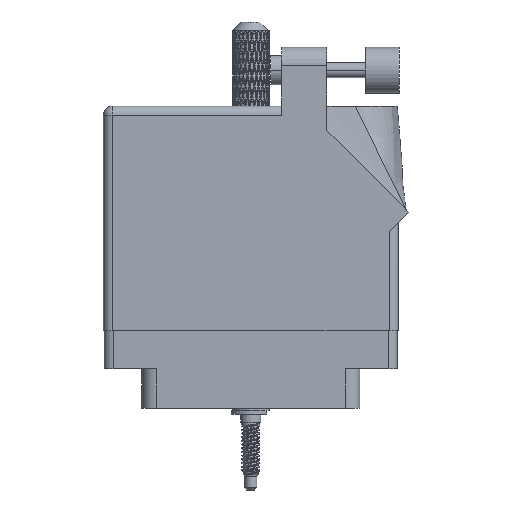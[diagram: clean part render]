
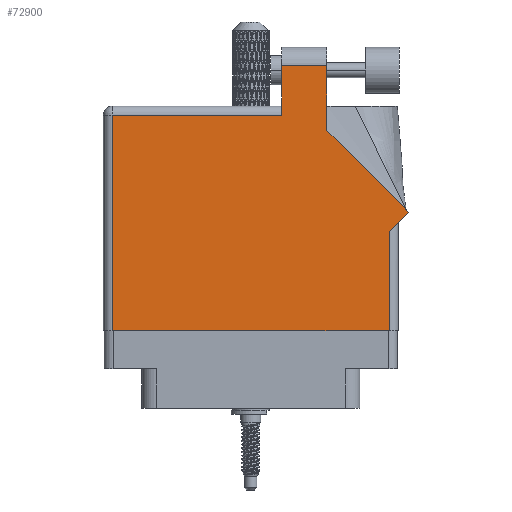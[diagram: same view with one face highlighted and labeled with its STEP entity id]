
A CAD part, front view. The second image highlights one B-rep face of the part: STEP entity #72900.
In plain terms, the highlighted face is planar.
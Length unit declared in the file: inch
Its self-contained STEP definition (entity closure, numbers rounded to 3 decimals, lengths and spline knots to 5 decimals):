
#236 = ORIENTED_EDGE ( 'NONE', *, *, #58033, .T. ) ;
#640 = CARTESIAN_POINT ( 'NONE',  ( 0., 0., 0. ) ) ;
#4222 = DIRECTION ( 'NONE',  ( -1., 0., 0. ) ) ;
#5205 = EDGE_CURVE ( 'NONE', #50115, #17018, #53685, .T. ) ;
#7064 = DIRECTION ( 'NONE',  ( 0., -1., 0. ) ) ;
#10006 = VERTEX_POINT ( 'NONE', #33152 ) ;
#10097 = LINE ( 'NONE', #22902, #75804 ) ;
#12381 = CARTESIAN_POINT ( 'NONE',  ( 1.217, 1.53, 0. ) ) ;
#14706 = VECTOR ( 'NONE', #36024, 39.37008 ) ;
#17018 = VERTEX_POINT ( 'NONE', #50581 ) ;
#19687 = FACE_OUTER_BOUND ( 'NONE', #66685, .T. ) ;
#21158 = CARTESIAN_POINT ( 'NONE',  ( 1.948, 0., 0. ) ) ;
#22902 = CARTESIAN_POINT ( 'NONE',  ( 2.08071, 0.80771, 0. ) ) ;
#23460 = DIRECTION ( 'NONE',  ( -1., 0., 0. ) ) ;
#24929 = EDGE_CURVE ( 'NONE', #10006, #38995, #44352, .T. ) ;
#25370 = VECTOR ( 'NONE', #62608, 39.37008 ) ;
#27341 = VECTOR ( 'NONE', #70199, 39.37008 ) ;
#27861 = ORIENTED_EDGE ( 'NONE', *, *, #32482, .T. ) ;
#28465 = VECTOR ( 'NONE', #41269, 39.37008 ) ;
#29654 = VECTOR ( 'NONE', #30847, 39.37008 ) ;
#30813 = CARTESIAN_POINT ( 'NONE',  ( 1.524, 1.36442, 0. ) ) ;
#30847 = DIRECTION ( 'NONE',  ( 0., -1., 0. ) ) ;
#31731 = VERTEX_POINT ( 'NONE', #30813 ) ;
#31972 = VERTEX_POINT ( 'NONE', #21158 ) ;
#32482 = EDGE_CURVE ( 'NONE', #38995, #51647, #56055, .T. ) ;
#33152 = CARTESIAN_POINT ( 'NONE',  ( 1.524, 1.805, 0. ) ) ;
#35277 = LINE ( 'NONE', #640, #40341 ) ;
#36024 = DIRECTION ( 'NONE',  ( 0., 1., 0. ) ) ;
#38915 = CARTESIAN_POINT ( 'NONE',  ( 1.217, 1.805, 0. ) ) ;
#38995 = VERTEX_POINT ( 'NONE', #38915 ) ;
#39507 = VERTEX_POINT ( 'NONE', #71466 ) ;
#39673 = ORIENTED_EDGE ( 'NONE', *, *, #86733, .T. ) ;
#40341 = VECTOR ( 'NONE', #48051, 39.37008 ) ;
#41269 = DIRECTION ( 'NONE',  ( 0.707, 0.707, 0. ) ) ;
#42378 = EDGE_CURVE ( 'NONE', #77909, #39507, #66337, .T. ) ;
#44352 = LINE ( 'NONE', #102861, #25370 ) ;
#45920 = VECTOR ( 'NONE', #7064, 39.37008 ) ;
#45976 = ORIENTED_EDGE ( 'NONE', *, *, #98456, .T. ) ;
#48051 = DIRECTION ( 'NONE',  ( 1., 0., 0. ) ) ;
#50115 = VERTEX_POINT ( 'NONE', #103552 ) ;
#50314 = EDGE_CURVE ( 'NONE', #51647, #50115, #90576, .T. ) ;
#50581 = CARTESIAN_POINT ( 'NONE',  ( 0.062, 0., 0. ) ) ;
#51647 = VERTEX_POINT ( 'NONE', #53913 ) ;
#53015 = DIRECTION ( 'NONE',  ( 0., 0., -1. ) ) ;
#53289 = CARTESIAN_POINT ( 'NONE',  ( 1.948, 0.737, 0. ) ) ;
#53357 = PLANE ( 'NONE',  #101608 ) ;
#53685 = LINE ( 'NONE', #94021, #29654 ) ;
#53913 = CARTESIAN_POINT ( 'NONE',  ( 1.217, 1.468, 0. ) ) ;
#56055 = LINE ( 'NONE', #12381, #45920 ) ;
#57109 = CARTESIAN_POINT ( 'NONE',  ( 2.01, 0.737, 0. ) ) ;
#58033 = EDGE_CURVE ( 'NONE', #39507, #31731, #10097, .T. ) ;
#62608 = DIRECTION ( 'NONE',  ( -1., 0., 0. ) ) ;
#64051 = VECTOR ( 'NONE', #23460, 39.37008 ) ;
#66337 = LINE ( 'NONE', #57109, #28465 ) ;
#66647 = ORIENTED_EDGE ( 'NONE', *, *, #83981, .T. ) ;
#66685 = EDGE_LOOP ( 'NONE', ( #45976, #99553, #27861, #69992, #87516, #66647, #39673, #98774, #236 ) ) ;
#69178 = CARTESIAN_POINT ( 'NONE',  ( 0., 1.53, 0. ) ) ;
#69992 = ORIENTED_EDGE ( 'NONE', *, *, #50314, .T. ) ;
#70199 = DIRECTION ( 'NONE',  ( 0., 1., 0. ) ) ;
#71466 = CARTESIAN_POINT ( 'NONE',  ( 2.08071, 0.80771, 0. ) ) ;
#72900 = ADVANCED_FACE ( 'NONE', ( #19687 ), #53357, .F. ) ;
#75804 = VECTOR ( 'NONE', #103085, 39.37008 ) ;
#76556 = LINE ( 'NONE', #94919, #27341 ) ;
#77909 = VERTEX_POINT ( 'NONE', #88079 ) ;
#80294 = CARTESIAN_POINT ( 'NONE',  ( 0., 1.468, 0. ) ) ;
#83981 = EDGE_CURVE ( 'NONE', #17018, #31972, #35277, .T. ) ;
#86733 = EDGE_CURVE ( 'NONE', #31972, #77909, #91850, .T. ) ;
#87516 = ORIENTED_EDGE ( 'NONE', *, *, #5205, .T. ) ;
#88079 = CARTESIAN_POINT ( 'NONE',  ( 1.948, 0.675, 0. ) ) ;
#90576 = LINE ( 'NONE', #80294, #64051 ) ;
#91850 = LINE ( 'NONE', #53289, #14706 ) ;
#94021 = CARTESIAN_POINT ( 'NONE',  ( 0.062, 0., 0. ) ) ;
#94919 = CARTESIAN_POINT ( 'NONE',  ( 1.524, 1.36442, 0. ) ) ;
#98456 = EDGE_CURVE ( 'NONE', #31731, #10006, #76556, .T. ) ;
#98774 = ORIENTED_EDGE ( 'NONE', *, *, #42378, .T. ) ;
#99553 = ORIENTED_EDGE ( 'NONE', *, *, #24929, .T. ) ;
#101608 = AXIS2_PLACEMENT_3D ( 'NONE', #69178, #53015, #4222 ) ;
#102861 = CARTESIAN_POINT ( 'NONE',  ( 1.217, 1.805, 0. ) ) ;
#103085 = DIRECTION ( 'NONE',  ( -0.707, 0.707, 0. ) ) ;
#103552 = CARTESIAN_POINT ( 'NONE',  ( 0.062, 1.468, 0. ) ) ;
